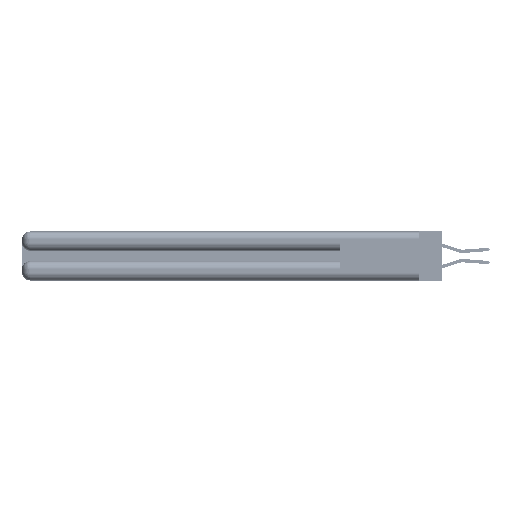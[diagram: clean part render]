
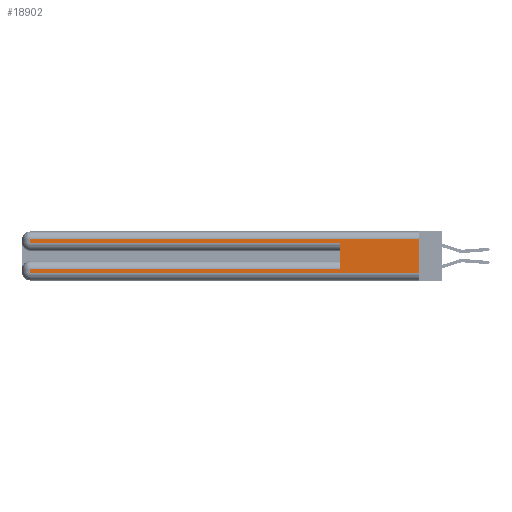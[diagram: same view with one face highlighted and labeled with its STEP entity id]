
A CAD part, left-side view. The second image highlights one B-rep face of the part: STEP entity #18902.
In plain terms, the highlighted planar face has unit normal (-1, 0, 0).
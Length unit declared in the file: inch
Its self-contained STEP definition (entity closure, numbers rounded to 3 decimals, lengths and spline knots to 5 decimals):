
#73 = EDGE_CURVE ( 'NONE', #13124, #46976, #50085, .T. ) ;
#610 = ORIENTED_EDGE ( 'NONE', *, *, #42534, .T. ) ;
#2011 = VERTEX_POINT ( 'NONE', #6593 ) ;
#2722 = PLANE ( 'NONE',  #45712 ) ;
#3978 = CARTESIAN_POINT ( 'NONE',  ( 0., 2.94, 0.37 ) ) ;
#4094 = ORIENTED_EDGE ( 'NONE', *, *, #23256, .T. ) ;
#4172 = CARTESIAN_POINT ( 'NONE',  ( 0., 2.94, 0.285 ) ) ;
#4828 = DIRECTION ( 'NONE',  ( 0., 1., 0. ) ) ;
#5025 = LINE ( 'NONE', #9978, #42840 ) ;
#5703 = VECTOR ( 'NONE', #51343, 39.37008 ) ;
#6197 = LINE ( 'NONE', #32353, #13669 ) ;
#6593 = CARTESIAN_POINT ( 'NONE',  ( 0., 2.94, 0.06 ) ) ;
#6954 = EDGE_CURVE ( 'NONE', #37005, #21884, #42752, .T. ) ;
#7009 = DIRECTION ( 'NONE',  ( 0., 1., 0. ) ) ;
#7979 = VERTEX_POINT ( 'NONE', #8551 ) ;
#8551 = CARTESIAN_POINT ( 'NONE',  ( 0., 0., 0.31 ) ) ;
#8654 = VECTOR ( 'NONE', #49302, 39.37008 ) ;
#9978 = CARTESIAN_POINT ( 'NONE',  ( 0., 0., 0.37 ) ) ;
#10165 = LINE ( 'NONE', #12673, #33035 ) ;
#10173 = EDGE_CURVE ( 'NONE', #7979, #10545, #5025, .T. ) ;
#10545 = VERTEX_POINT ( 'NONE', #20889 ) ;
#12175 = FACE_OUTER_BOUND ( 'NONE', #19988, .T. ) ;
#12508 = DIRECTION ( 'NONE',  ( 0., 0., -1. ) ) ;
#12523 = LINE ( 'NONE', #3978, #5703 ) ;
#12646 = CARTESIAN_POINT ( 'NONE',  ( 0., 0.6, 0.145 ) ) ;
#12673 = CARTESIAN_POINT ( 'NONE',  ( 0., 2.94, 0.37 ) ) ;
#12678 = DIRECTION ( 'NONE',  ( 0., -1., 0. ) ) ;
#12985 = ORIENTED_EDGE ( 'NONE', *, *, #73, .T. ) ;
#13124 = VERTEX_POINT ( 'NONE', #34270 ) ;
#13573 = EDGE_CURVE ( 'NONE', #13124, #21884, #40759, .T. ) ;
#13643 = DIRECTION ( 'NONE',  ( 0., 0., -1. ) ) ;
#13669 = VECTOR ( 'NONE', #4828, 39.37008 ) ;
#15991 = ORIENTED_EDGE ( 'NONE', *, *, #20662, .T. ) ;
#17418 = CARTESIAN_POINT ( 'NONE',  ( 0., 0., 0.285 ) ) ;
#18902 = ADVANCED_FACE ( 'NONE', ( #12175 ), #2722, .F. ) ;
#19542 = DIRECTION ( 'NONE',  ( 0., 0., -1. ) ) ;
#19988 = EDGE_LOOP ( 'NONE', ( #34099, #4094, #15991, #37051, #44999, #12985, #26485, #610 ) ) ;
#20662 = EDGE_CURVE ( 'NONE', #28163, #37005, #10165, .T. ) ;
#20889 = CARTESIAN_POINT ( 'NONE',  ( 0., 0., 0.06 ) ) ;
#21307 = LINE ( 'NONE', #24580, #33028 ) ;
#21481 = EDGE_CURVE ( 'NONE', #46976, #2011, #12523, .T. ) ;
#21884 = VERTEX_POINT ( 'NONE', #28516 ) ;
#23256 = EDGE_CURVE ( 'NONE', #7979, #28163, #6197, .T. ) ;
#23369 = VECTOR ( 'NONE', #7009, 39.37008 ) ;
#24580 = CARTESIAN_POINT ( 'NONE',  ( 0., 0., 0.06 ) ) ;
#24902 = DIRECTION ( 'NONE',  ( 0., 0., 1. ) ) ;
#26485 = ORIENTED_EDGE ( 'NONE', *, *, #21481, .T. ) ;
#28070 = CARTESIAN_POINT ( 'NONE',  ( 0., 2.94, 0.085 ) ) ;
#28163 = VERTEX_POINT ( 'NONE', #39186 ) ;
#28516 = CARTESIAN_POINT ( 'NONE',  ( 0., 0.6, 0.285 ) ) ;
#32353 = CARTESIAN_POINT ( 'NONE',  ( 0., 0., 0.31 ) ) ;
#33028 = VECTOR ( 'NONE', #12678, 39.37008 ) ;
#33035 = VECTOR ( 'NONE', #12508, 39.37008 ) ;
#34099 = ORIENTED_EDGE ( 'NONE', *, *, #10173, .F. ) ;
#34270 = CARTESIAN_POINT ( 'NONE',  ( 0., 0.6, 0.085 ) ) ;
#37005 = VERTEX_POINT ( 'NONE', #4172 ) ;
#37051 = ORIENTED_EDGE ( 'NONE', *, *, #6954, .T. ) ;
#38271 = VECTOR ( 'NONE', #24902, 39.37008 ) ;
#39186 = CARTESIAN_POINT ( 'NONE',  ( 0., 2.94, 0.31 ) ) ;
#40759 = LINE ( 'NONE', #12646, #38271 ) ;
#42534 = EDGE_CURVE ( 'NONE', #2011, #10545, #21307, .T. ) ;
#42752 = LINE ( 'NONE', #17418, #8654 ) ;
#42840 = VECTOR ( 'NONE', #13643, 39.37008 ) ;
#44999 = ORIENTED_EDGE ( 'NONE', *, *, #13573, .F. ) ;
#45712 = AXIS2_PLACEMENT_3D ( 'NONE', #50441, #46597, #19542 ) ;
#46597 = DIRECTION ( 'NONE',  ( 1., 0., 0. ) ) ;
#46976 = VERTEX_POINT ( 'NONE', #28070 ) ;
#49302 = DIRECTION ( 'NONE',  ( 0., -1., 0. ) ) ;
#50010 = CARTESIAN_POINT ( 'NONE',  ( 0., 0., 0.085 ) ) ;
#50085 = LINE ( 'NONE', #50010, #23369 ) ;
#50441 = CARTESIAN_POINT ( 'NONE',  ( 0., 0., 0.37 ) ) ;
#51343 = DIRECTION ( 'NONE',  ( 0., 0., -1. ) ) ;
